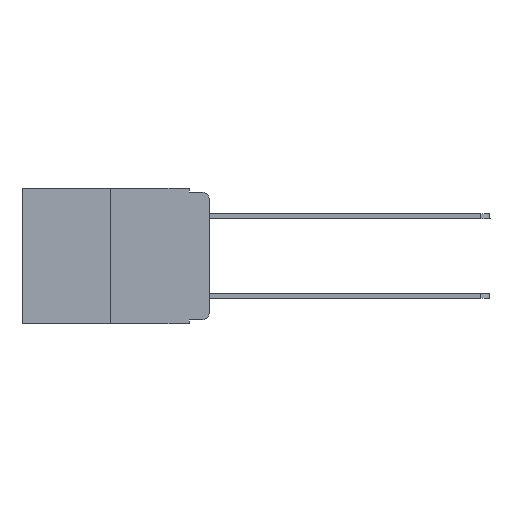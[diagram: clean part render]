
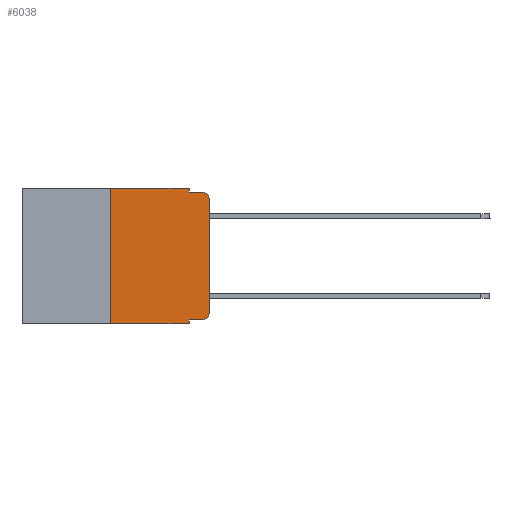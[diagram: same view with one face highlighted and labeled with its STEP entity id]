
A CAD part, left-side view. The second image highlights one B-rep face of the part: STEP entity #6038.
In plain terms, the highlighted planar face has unit normal (-1, 0, 0).
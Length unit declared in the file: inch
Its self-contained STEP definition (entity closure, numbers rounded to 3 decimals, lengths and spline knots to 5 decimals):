
#89 = ORIENTED_EDGE ( 'NONE', *, *, #9495, .T. ) ;
#326 = VECTOR ( 'NONE', #1783, 39.37008 ) ;
#347 = CARTESIAN_POINT ( 'NONE',  ( 0., 0.02, -0.333 ) ) ;
#454 = LINE ( 'NONE', #8408, #4871 ) ;
#579 = DIRECTION ( 'NONE',  ( 0., 0., -1. ) ) ;
#582 = ORIENTED_EDGE ( 'NONE', *, *, #9863, .F. ) ;
#668 = DIRECTION ( 'NONE',  ( 0., 0., -1. ) ) ;
#734 = DIRECTION ( 'NONE',  ( -1., 0., 0. ) ) ;
#746 = VERTEX_POINT ( 'NONE', #7132 ) ;
#835 = ORIENTED_EDGE ( 'NONE', *, *, #3437, .T. ) ;
#1019 = VECTOR ( 'NONE', #4939, 39.37008 ) ;
#1184 = ORIENTED_EDGE ( 'NONE', *, *, #2906, .T. ) ;
#1278 = CARTESIAN_POINT ( 'NONE',  ( 0., 0.25, 0. ) ) ;
#1434 = LINE ( 'NONE', #4324, #6109 ) ;
#1624 = CARTESIAN_POINT ( 'NONE',  ( 0., 0.02, -0.03 ) ) ;
#1629 = CARTESIAN_POINT ( 'NONE',  ( 0., 0.473, 0. ) ) ;
#1783 = DIRECTION ( 'NONE',  ( 0., 0., -1. ) ) ;
#2155 = ORIENTED_EDGE ( 'NONE', *, *, #12075, .T. ) ;
#2248 = CARTESIAN_POINT ( 'NONE',  ( 0., 0.051, -0.01 ) ) ;
#2320 = CARTESIAN_POINT ( 'NONE',  ( 0., 0., -0.313 ) ) ;
#2744 = LINE ( 'NONE', #8582, #326 ) ;
#2788 = AXIS2_PLACEMENT_3D ( 'NONE', #1624, #734, #668 ) ;
#2833 = EDGE_CURVE ( 'NONE', #7525, #6190, #6583, .T. ) ;
#2845 = CARTESIAN_POINT ( 'NONE',  ( 0., 0., 0. ) ) ;
#2906 = EDGE_CURVE ( 'NONE', #10297, #6064, #9247, .T. ) ;
#3309 = DIRECTION ( 'NONE',  ( 0., -1., 0. ) ) ;
#3433 = FACE_OUTER_BOUND ( 'NONE', #12742, .T. ) ;
#3437 = EDGE_CURVE ( 'NONE', #7315, #7525, #454, .T. ) ;
#3808 = ORIENTED_EDGE ( 'NONE', *, *, #5299, .F. ) ;
#4005 = ORIENTED_EDGE ( 'NONE', *, *, #8540, .F. ) ;
#4309 = ORIENTED_EDGE ( 'NONE', *, *, #10166, .F. ) ;
#4324 = CARTESIAN_POINT ( 'NONE',  ( 0., 0.473, 0. ) ) ;
#4736 = VERTEX_POINT ( 'NONE', #5417 ) ;
#4871 = VECTOR ( 'NONE', #12383, 39.37008 ) ;
#4939 = DIRECTION ( 'NONE',  ( 0., -1., 0. ) ) ;
#4956 = VERTEX_POINT ( 'NONE', #2248 ) ;
#5299 = EDGE_CURVE ( 'NONE', #746, #6214, #9625, .T. ) ;
#5417 = CARTESIAN_POINT ( 'NONE',  ( 0., 0.051, -0.343 ) ) ;
#5421 = CARTESIAN_POINT ( 'NONE',  ( 0., 0.473, -0.343 ) ) ;
#5422 = VERTEX_POINT ( 'NONE', #6250 ) ;
#5565 = DIRECTION ( 'NONE',  ( 1., 0., 0. ) ) ;
#5638 = VECTOR ( 'NONE', #12634, 39.37008 ) ;
#5813 = LINE ( 'NONE', #2845, #6584 ) ;
#5950 = DIRECTION ( 'NONE',  ( 0., 0., 1. ) ) ;
#6038 = ADVANCED_FACE ( 'NONE', ( #3433 ), #10505, .F. ) ;
#6064 = VERTEX_POINT ( 'NONE', #9260 ) ;
#6105 = CARTESIAN_POINT ( 'NONE',  ( 0., 0.02, -0.313 ) ) ;
#6109 = VECTOR ( 'NONE', #3309, 39.37008 ) ;
#6190 = VERTEX_POINT ( 'NONE', #2320 ) ;
#6214 = VERTEX_POINT ( 'NONE', #1278 ) ;
#6250 = CARTESIAN_POINT ( 'NONE',  ( 0., 0.051, 0. ) ) ;
#6336 = CARTESIAN_POINT ( 'NONE',  ( 0., 0.051, 0. ) ) ;
#6358 = DIRECTION ( 'NONE',  ( 0., 0., -1. ) ) ;
#6583 = CIRCLE ( 'NONE', #7627, 0.02 ) ;
#6584 = VECTOR ( 'NONE', #5950, 39.37008 ) ;
#7132 = CARTESIAN_POINT ( 'NONE',  ( 0., 0.25, -0.343 ) ) ;
#7315 = VERTEX_POINT ( 'NONE', #9533 ) ;
#7525 = VERTEX_POINT ( 'NONE', #347 ) ;
#7578 = LINE ( 'NONE', #5421, #11263 ) ;
#7627 = AXIS2_PLACEMENT_3D ( 'NONE', #6105, #9129, #6358 ) ;
#8408 = CARTESIAN_POINT ( 'NONE',  ( 0., 0.051, -0.333 ) ) ;
#8540 = EDGE_CURVE ( 'NONE', #7315, #4736, #2744, .T. ) ;
#8582 = CARTESIAN_POINT ( 'NONE',  ( 0., 0.051, 0. ) ) ;
#8661 = CARTESIAN_POINT ( 'NONE',  ( 0., 0.25, 0. ) ) ;
#9016 = ORIENTED_EDGE ( 'NONE', *, *, #2833, .T. ) ;
#9129 = DIRECTION ( 'NONE',  ( -1., 0., 0. ) ) ;
#9247 = CIRCLE ( 'NONE', #2788, 0.02 ) ;
#9260 = CARTESIAN_POINT ( 'NONE',  ( 0., 0.02, -0.01 ) ) ;
#9495 = EDGE_CURVE ( 'NONE', #746, #4736, #7578, .T. ) ;
#9525 = DIRECTION ( 'NONE',  ( 0., 0., -1. ) ) ;
#9533 = CARTESIAN_POINT ( 'NONE',  ( 0., 0.051, -0.333 ) ) ;
#9625 = LINE ( 'NONE', #8661, #5638 ) ;
#9863 = EDGE_CURVE ( 'NONE', #5422, #4956, #11325, .T. ) ;
#10166 = EDGE_CURVE ( 'NONE', #6214, #5422, #1434, .T. ) ;
#10297 = VERTEX_POINT ( 'NONE', #12537 ) ;
#10395 = AXIS2_PLACEMENT_3D ( 'NONE', #1629, #5565, #9525 ) ;
#10414 = DIRECTION ( 'NONE',  ( 0., -1., 0. ) ) ;
#10433 = ORIENTED_EDGE ( 'NONE', *, *, #12607, .F. ) ;
#10505 = PLANE ( 'NONE',  #10395 ) ;
#11101 = CARTESIAN_POINT ( 'NONE',  ( 0., 0.051, -0.01 ) ) ;
#11161 = LINE ( 'NONE', #11101, #1019 ) ;
#11263 = VECTOR ( 'NONE', #10414, 39.37008 ) ;
#11325 = LINE ( 'NONE', #6336, #12750 ) ;
#12075 = EDGE_CURVE ( 'NONE', #6190, #10297, #5813, .T. ) ;
#12383 = DIRECTION ( 'NONE',  ( 0., -1., 0. ) ) ;
#12537 = CARTESIAN_POINT ( 'NONE',  ( 0., 0., -0.03 ) ) ;
#12607 = EDGE_CURVE ( 'NONE', #4956, #6064, #11161, .T. ) ;
#12634 = DIRECTION ( 'NONE',  ( 0., 0., 1. ) ) ;
#12742 = EDGE_LOOP ( 'NONE', ( #2155, #1184, #10433, #582, #4309, #3808, #89, #4005, #835, #9016 ) ) ;
#12750 = VECTOR ( 'NONE', #579, 39.37008 ) ;
